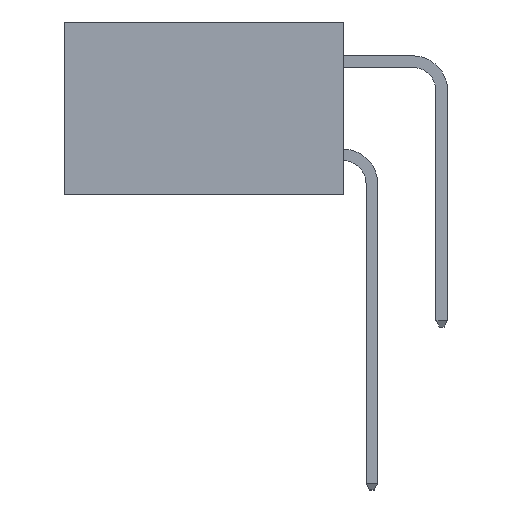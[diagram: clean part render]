
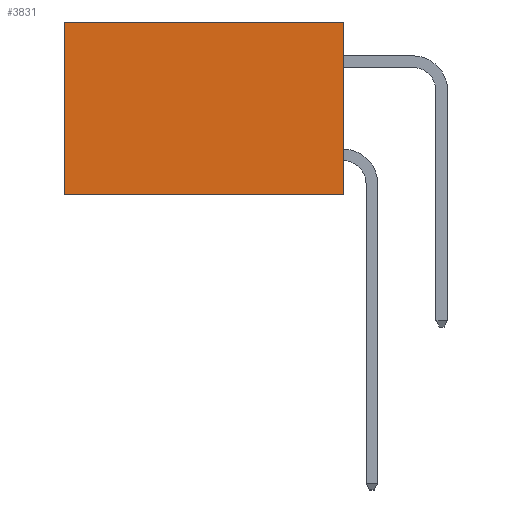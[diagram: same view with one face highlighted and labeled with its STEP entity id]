
A CAD part, left-side view. The second image highlights one B-rep face of the part: STEP entity #3831.
In plain terms, the highlighted planar face has unit normal (-1, 0, 0).
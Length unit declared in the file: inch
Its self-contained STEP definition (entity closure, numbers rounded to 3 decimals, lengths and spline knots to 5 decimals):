
#102 = EDGE_CURVE ( 'NONE', #6136, #7305, #12863, .T. ) ;
#330 = CARTESIAN_POINT ( 'NONE',  ( 0.2615, 0., 0. ) ) ;
#885 = FACE_OUTER_BOUND ( 'NONE', #10321, .T. ) ;
#1415 = EDGE_CURVE ( 'NONE', #11047, #12650, #3545, .T. ) ;
#1686 = CARTESIAN_POINT ( 'NONE',  ( 0.2615, 0., 0. ) ) ;
#2191 = EDGE_CURVE ( 'NONE', #11047, #6136, #12829, .T. ) ;
#3156 = ORIENTED_EDGE ( 'NONE', *, *, #102, .T. ) ;
#3545 = LINE ( 'NONE', #7034, #8585 ) ;
#3630 = DIRECTION ( 'NONE',  ( 0., 1., 0. ) ) ;
#3644 = CARTESIAN_POINT ( 'NONE',  ( 0.2615, 0., -0.37 ) ) ;
#3831 = ADVANCED_FACE ( 'NONE', ( #885 ), #12934, .F. ) ;
#4503 = VECTOR ( 'NONE', #13046, 39.37008 ) ;
#4684 = ORIENTED_EDGE ( 'NONE', *, *, #1415, .F. ) ;
#5054 = ORIENTED_EDGE ( 'NONE', *, *, #7624, .F. ) ;
#6136 = VERTEX_POINT ( 'NONE', #8850 ) ;
#6665 = AXIS2_PLACEMENT_3D ( 'NONE', #12966, #12923, #12920 ) ;
#6678 = CARTESIAN_POINT ( 'NONE',  ( 0.2615, 0.6, -0.37 ) ) ;
#7034 = CARTESIAN_POINT ( 'NONE',  ( 0.2615, 0., -0.37 ) ) ;
#7187 = DIRECTION ( 'NONE',  ( 0., 0., -1. ) ) ;
#7305 = VERTEX_POINT ( 'NONE', #6678 ) ;
#7624 = EDGE_CURVE ( 'NONE', #12650, #7305, #10180, .T. ) ;
#8297 = CARTESIAN_POINT ( 'NONE',  ( 0.2615, 0., -0.37 ) ) ;
#8585 = VECTOR ( 'NONE', #7187, 39.37008 ) ;
#8850 = CARTESIAN_POINT ( 'NONE',  ( 0.2615, 0.6, 0. ) ) ;
#9197 = DIRECTION ( 'NONE',  ( 0., 1., 0. ) ) ;
#10138 = VECTOR ( 'NONE', #9197, 39.37008 ) ;
#10180 = LINE ( 'NONE', #3644, #12864 ) ;
#10321 = EDGE_LOOP ( 'NONE', ( #3156, #5054, #4684, #10666 ) ) ;
#10666 = ORIENTED_EDGE ( 'NONE', *, *, #2191, .T. ) ;
#11047 = VERTEX_POINT ( 'NONE', #1686 ) ;
#12650 = VERTEX_POINT ( 'NONE', #8297 ) ;
#12829 = LINE ( 'NONE', #330, #10138 ) ;
#12863 = LINE ( 'NONE', #13108, #4503 ) ;
#12864 = VECTOR ( 'NONE', #3630, 39.37008 ) ;
#12920 = DIRECTION ( 'NONE',  ( 0., 0., -1. ) ) ;
#12923 = DIRECTION ( 'NONE',  ( 1., 0., 0. ) ) ;
#12934 = PLANE ( 'NONE',  #6665 ) ;
#12966 = CARTESIAN_POINT ( 'NONE',  ( 0.2615, 0., -0.37 ) ) ;
#13046 = DIRECTION ( 'NONE',  ( 0., 0., -1. ) ) ;
#13108 = CARTESIAN_POINT ( 'NONE',  ( 0.2615, 0.6, -0.37 ) ) ;
